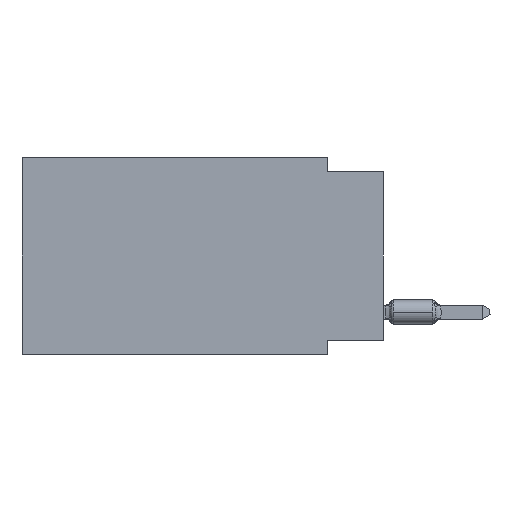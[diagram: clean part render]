
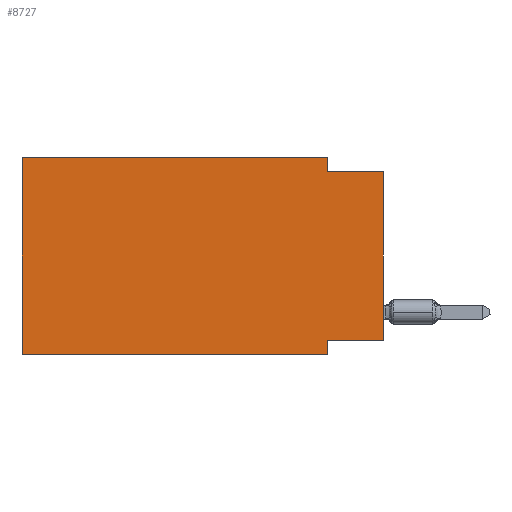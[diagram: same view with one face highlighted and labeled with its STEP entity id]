
A CAD part, left-side view. The second image highlights one B-rep face of the part: STEP entity #8727.
In plain terms, the highlighted planar face has unit normal (-1, 0, 0).
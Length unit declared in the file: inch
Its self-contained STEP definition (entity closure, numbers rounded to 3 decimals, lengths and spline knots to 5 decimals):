
#110 = VECTOR ( 'NONE', #28957, 39.37008 ) ;
#391 = CARTESIAN_POINT ( 'NONE',  ( 0., 0.1, -0.35 ) ) ;
#623 = CARTESIAN_POINT ( 'NONE',  ( 0., 0.1, 0. ) ) ;
#924 = DIRECTION ( 'NONE',  ( 0., -1., 0. ) ) ;
#1003 = EDGE_CURVE ( 'NONE', #10158, #28677, #17073, .T. ) ;
#1274 = EDGE_LOOP ( 'NONE', ( #20809, #3425, #33734, #1533, #17979, #2818, #28955, #4047 ) ) ;
#1533 = ORIENTED_EDGE ( 'NONE', *, *, #11863, .F. ) ;
#1775 = CARTESIAN_POINT ( 'NONE',  ( 0., 0., -0.025 ) ) ;
#1953 = LINE ( 'NONE', #1775, #110 ) ;
#2720 = FACE_OUTER_BOUND ( 'NONE', #1274, .T. ) ;
#2818 = ORIENTED_EDGE ( 'NONE', *, *, #20105, .T. ) ;
#2979 = VERTEX_POINT ( 'NONE', #19575 ) ;
#3425 = ORIENTED_EDGE ( 'NONE', *, *, #12591, .F. ) ;
#3585 = VECTOR ( 'NONE', #26645, 39.37008 ) ;
#3969 = CARTESIAN_POINT ( 'NONE',  ( 0., 0.1, -0.35 ) ) ;
#4047 = ORIENTED_EDGE ( 'NONE', *, *, #21908, .F. ) ;
#7549 = CARTESIAN_POINT ( 'NONE',  ( 0., 0.645, -0.35 ) ) ;
#7803 = VECTOR ( 'NONE', #924, 39.37008 ) ;
#8727 = ADVANCED_FACE ( 'NONE', ( #2720 ), #32386, .F. ) ;
#9873 = DIRECTION ( 'NONE',  ( 0., -1., 0. ) ) ;
#9910 = EDGE_CURVE ( 'NONE', #27635, #15867, #27063, .T. ) ;
#10158 = VERTEX_POINT ( 'NONE', #7549 ) ;
#11575 = EDGE_CURVE ( 'NONE', #2979, #16665, #13495, .T. ) ;
#11863 = EDGE_CURVE ( 'NONE', #28677, #21298, #18043, .T. ) ;
#12308 = AXIS2_PLACEMENT_3D ( 'NONE', #29730, #24392, #13546 ) ;
#12591 = EDGE_CURVE ( 'NONE', #32712, #16665, #1953, .T. ) ;
#13307 = CARTESIAN_POINT ( 'NONE',  ( 0., 0., -0.325 ) ) ;
#13495 = LINE ( 'NONE', #31987, #3585 ) ;
#13546 = DIRECTION ( 'NONE',  ( 0., 0., -1. ) ) ;
#14427 = LINE ( 'NONE', #25261, #7803 ) ;
#15867 = VERTEX_POINT ( 'NONE', #3969 ) ;
#16062 = VECTOR ( 'NONE', #20080, 39.37008 ) ;
#16665 = VERTEX_POINT ( 'NONE', #22720 ) ;
#16733 = DIRECTION ( 'NONE',  ( 0., 0., -1. ) ) ;
#17073 = LINE ( 'NONE', #27565, #33669 ) ;
#17979 = ORIENTED_EDGE ( 'NONE', *, *, #1003, .F. ) ;
#18043 = LINE ( 'NONE', #29229, #26284 ) ;
#19575 = CARTESIAN_POINT ( 'NONE',  ( 0., 0., -0.325 ) ) ;
#19752 = DIRECTION ( 'NONE',  ( 0., 0., 1. ) ) ;
#19902 = LINE ( 'NONE', #30736, #16062 ) ;
#20080 = DIRECTION ( 'NONE',  ( 0., 0., -1. ) ) ;
#20105 = EDGE_CURVE ( 'NONE', #10158, #15867, #14427, .T. ) ;
#20809 = ORIENTED_EDGE ( 'NONE', *, *, #11575, .T. ) ;
#21298 = VERTEX_POINT ( 'NONE', #623 ) ;
#21301 = DIRECTION ( 'NONE',  ( 0., 1., 0. ) ) ;
#21400 = CARTESIAN_POINT ( 'NONE',  ( 0., 0.1, -0.025 ) ) ;
#21908 = EDGE_CURVE ( 'NONE', #2979, #27635, #26810, .T. ) ;
#22420 = CARTESIAN_POINT ( 'NONE',  ( 0., 0.1, -0.325 ) ) ;
#22720 = CARTESIAN_POINT ( 'NONE',  ( 0., 0., -0.025 ) ) ;
#23758 = VECTOR ( 'NONE', #21301, 39.37008 ) ;
#24392 = DIRECTION ( 'NONE',  ( 1., 0., 0. ) ) ;
#25261 = CARTESIAN_POINT ( 'NONE',  ( 0., 0.645, -0.35 ) ) ;
#26030 = CARTESIAN_POINT ( 'NONE',  ( 0., 0.645, 0. ) ) ;
#26284 = VECTOR ( 'NONE', #9873, 39.37008 ) ;
#26645 = DIRECTION ( 'NONE',  ( 0., 0., 1. ) ) ;
#26810 = LINE ( 'NONE', #13307, #23758 ) ;
#27063 = LINE ( 'NONE', #391, #27159 ) ;
#27159 = VECTOR ( 'NONE', #16733, 39.37008 ) ;
#27565 = CARTESIAN_POINT ( 'NONE',  ( 0., 0.645, 0. ) ) ;
#27635 = VERTEX_POINT ( 'NONE', #22420 ) ;
#28677 = VERTEX_POINT ( 'NONE', #26030 ) ;
#28955 = ORIENTED_EDGE ( 'NONE', *, *, #9910, .F. ) ;
#28957 = DIRECTION ( 'NONE',  ( 0., -1., 0. ) ) ;
#29229 = CARTESIAN_POINT ( 'NONE',  ( 0., 0.645, 0. ) ) ;
#29730 = CARTESIAN_POINT ( 'NONE',  ( 0., 0.645, 0. ) ) ;
#30736 = CARTESIAN_POINT ( 'NONE',  ( 0., 0.1, 0. ) ) ;
#31470 = EDGE_CURVE ( 'NONE', #21298, #32712, #19902, .T. ) ;
#31987 = CARTESIAN_POINT ( 'NONE',  ( 0., 0., 0. ) ) ;
#32386 = PLANE ( 'NONE',  #12308 ) ;
#32712 = VERTEX_POINT ( 'NONE', #21400 ) ;
#33669 = VECTOR ( 'NONE', #19752, 39.37008 ) ;
#33734 = ORIENTED_EDGE ( 'NONE', *, *, #31470, .F. ) ;
